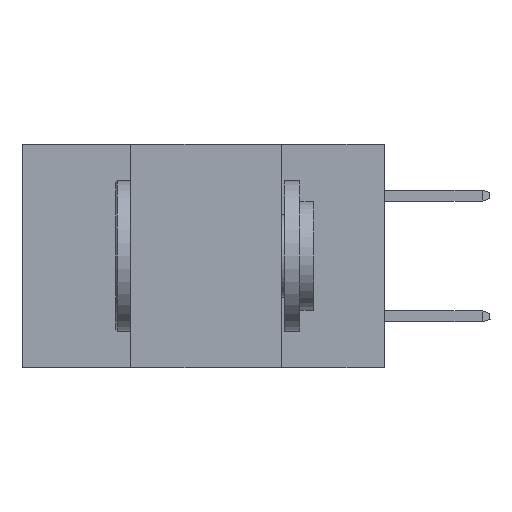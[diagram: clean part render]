
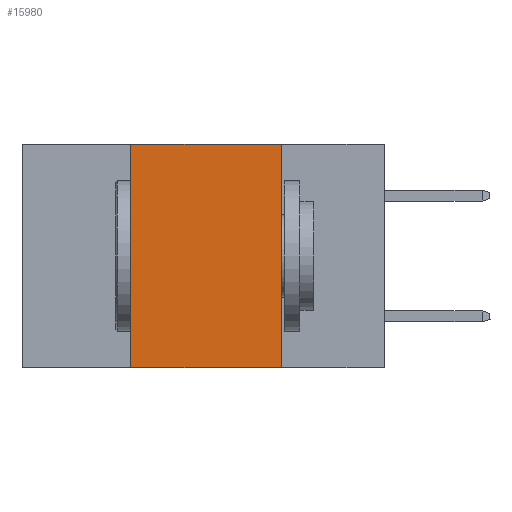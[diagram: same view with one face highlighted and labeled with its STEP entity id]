
A CAD part, left-side view. The second image highlights one B-rep face of the part: STEP entity #15980.
In plain terms, the highlighted planar face has unit normal (-1, 0, 0).
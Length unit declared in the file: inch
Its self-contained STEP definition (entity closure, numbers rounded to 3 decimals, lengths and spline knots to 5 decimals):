
#110 = ORIENTED_EDGE ( 'NONE', *, *, #16368, .T. ) ;
#884 = LINE ( 'NONE', #9079, #12257 ) ;
#1495 = EDGE_CURVE ( 'NONE', #2828, #12414, #884, .T. ) ;
#1643 = PLANE ( 'NONE',  #10266 ) ;
#1903 = CARTESIAN_POINT ( 'NONE',  ( 0., 0.42, -0.37 ) ) ;
#2710 = CARTESIAN_POINT ( 'NONE',  ( 0., 0.6, -0.37 ) ) ;
#2828 = VERTEX_POINT ( 'NONE', #13513 ) ;
#2884 = LINE ( 'NONE', #2710, #7299 ) ;
#3196 = LINE ( 'NONE', #8490, #14470 ) ;
#4644 = DIRECTION ( 'NONE',  ( 0., 0., 1. ) ) ;
#4682 = DIRECTION ( 'NONE',  ( 1., 0., 0. ) ) ;
#5083 = CARTESIAN_POINT ( 'NONE',  ( 0., 0.42, -0.37 ) ) ;
#5092 = EDGE_LOOP ( 'NONE', ( #15420, #17152, #10296, #110 ) ) ;
#6903 = EDGE_CURVE ( 'NONE', #14011, #2828, #12869, .T. ) ;
#7299 = VECTOR ( 'NONE', #13000, 39.37008 ) ;
#7320 = VERTEX_POINT ( 'NONE', #10844 ) ;
#8490 = CARTESIAN_POINT ( 'NONE',  ( 0., 0.17, -0.37 ) ) ;
#9079 = CARTESIAN_POINT ( 'NONE',  ( 0., 0.6, 0. ) ) ;
#9979 = DIRECTION ( 'NONE',  ( 0., 0., -1. ) ) ;
#10080 = DIRECTION ( 'NONE',  ( 0., -1., 0. ) ) ;
#10266 = AXIS2_PLACEMENT_3D ( 'NONE', #13447, #4682, #14926 ) ;
#10296 = ORIENTED_EDGE ( 'NONE', *, *, #6903, .F. ) ;
#10844 = CARTESIAN_POINT ( 'NONE',  ( 0., 0.17, -0.37 ) ) ;
#12006 = CARTESIAN_POINT ( 'NONE',  ( 0., 0.17, 0. ) ) ;
#12257 = VECTOR ( 'NONE', #10080, 39.37008 ) ;
#12410 = VECTOR ( 'NONE', #4644, 39.37008 ) ;
#12414 = VERTEX_POINT ( 'NONE', #12006 ) ;
#12869 = LINE ( 'NONE', #5083, #12410 ) ;
#13000 = DIRECTION ( 'NONE',  ( 0., -1., 0. ) ) ;
#13447 = CARTESIAN_POINT ( 'NONE',  ( 0., 0.6, 0. ) ) ;
#13513 = CARTESIAN_POINT ( 'NONE',  ( 0., 0.42, 0. ) ) ;
#13626 = EDGE_CURVE ( 'NONE', #12414, #7320, #3196, .T. ) ;
#14011 = VERTEX_POINT ( 'NONE', #1903 ) ;
#14470 = VECTOR ( 'NONE', #9979, 39.37008 ) ;
#14926 = DIRECTION ( 'NONE',  ( 0., 0., -1. ) ) ;
#15420 = ORIENTED_EDGE ( 'NONE', *, *, #13626, .F. ) ;
#15980 = ADVANCED_FACE ( 'NONE', ( #17154 ), #1643, .F. ) ;
#16368 = EDGE_CURVE ( 'NONE', #14011, #7320, #2884, .T. ) ;
#17152 = ORIENTED_EDGE ( 'NONE', *, *, #1495, .F. ) ;
#17154 = FACE_OUTER_BOUND ( 'NONE', #5092, .T. ) ;
